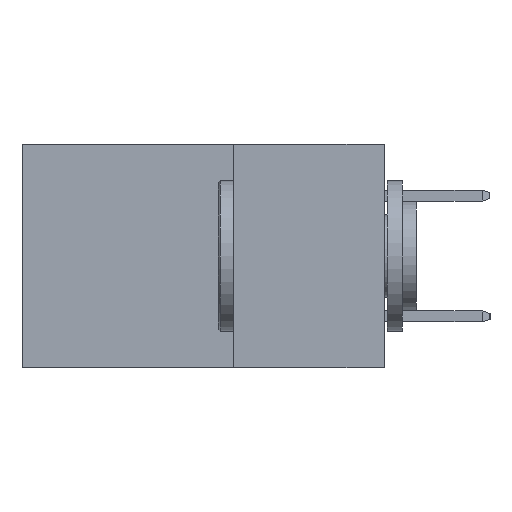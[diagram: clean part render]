
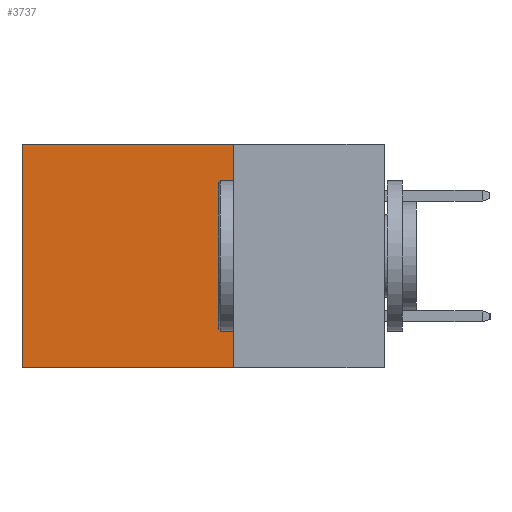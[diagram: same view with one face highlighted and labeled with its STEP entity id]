
A CAD part, left-side view. The second image highlights one B-rep face of the part: STEP entity #3737.
In plain terms, the highlighted planar face has unit normal (-1, 0, 0).
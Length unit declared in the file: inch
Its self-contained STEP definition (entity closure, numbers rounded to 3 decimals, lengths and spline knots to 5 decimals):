
#988 = EDGE_CURVE ( 'NONE', #3144, #2334, #13684, .T. ) ;
#1966 = EDGE_CURVE ( 'NONE', #3286, #10497, #11336, .T. ) ;
#2065 = VECTOR ( 'NONE', #4702, 39.37008 ) ;
#2334 = VERTEX_POINT ( 'NONE', #8466 ) ;
#2817 = FACE_OUTER_BOUND ( 'NONE', #7623, .T. ) ;
#3045 = DIRECTION ( 'NONE',  ( 0., 0., -1. ) ) ;
#3144 = VERTEX_POINT ( 'NONE', #10999 ) ;
#3286 = VERTEX_POINT ( 'NONE', #6830 ) ;
#3434 = CARTESIAN_POINT ( 'NONE',  ( 0.2615, 0.6, -0.37 ) ) ;
#3737 = ADVANCED_FACE ( 'NONE', ( #2817 ), #5657, .F. ) ;
#3754 = AXIS2_PLACEMENT_3D ( 'NONE', #6636, #5295, #5189 ) ;
#4532 = CARTESIAN_POINT ( 'NONE',  ( 0.2615, 0.25, 0. ) ) ;
#4702 = DIRECTION ( 'NONE',  ( 0., 1., 0. ) ) ;
#5082 = LINE ( 'NONE', #15346, #11401 ) ;
#5189 = DIRECTION ( 'NONE',  ( 0., 0., -1. ) ) ;
#5295 = DIRECTION ( 'NONE',  ( 1., 0., 0. ) ) ;
#5657 = PLANE ( 'NONE',  #3754 ) ;
#5928 = ORIENTED_EDGE ( 'NONE', *, *, #1966, .T. ) ;
#5994 = VECTOR ( 'NONE', #3045, 39.37008 ) ;
#6386 = EDGE_CURVE ( 'NONE', #10497, #2334, #9890, .T. ) ;
#6636 = CARTESIAN_POINT ( 'NONE',  ( 0.2615, 0.25, -0.37 ) ) ;
#6830 = CARTESIAN_POINT ( 'NONE',  ( 0.2615, 0.25, 0. ) ) ;
#7246 = CARTESIAN_POINT ( 'NONE',  ( 0.2615, 0.6, 0. ) ) ;
#7623 = EDGE_LOOP ( 'NONE', ( #9704, #14377, #8289, #5928 ) ) ;
#8035 = CARTESIAN_POINT ( 'NONE',  ( 0.2615, 0.25, -0.37 ) ) ;
#8289 = ORIENTED_EDGE ( 'NONE', *, *, #11616, .F. ) ;
#8439 = DIRECTION ( 'NONE',  ( 0., 1., 0. ) ) ;
#8466 = CARTESIAN_POINT ( 'NONE',  ( 0.2615, 0.6, -0.37 ) ) ;
#9704 = ORIENTED_EDGE ( 'NONE', *, *, #6386, .T. ) ;
#9890 = LINE ( 'NONE', #3434, #5994 ) ;
#10497 = VERTEX_POINT ( 'NONE', #7246 ) ;
#10618 = VECTOR ( 'NONE', #8439, 39.37008 ) ;
#10999 = CARTESIAN_POINT ( 'NONE',  ( 0.2615, 0.25, -0.37 ) ) ;
#11336 = LINE ( 'NONE', #4532, #2065 ) ;
#11401 = VECTOR ( 'NONE', #15258, 39.37008 ) ;
#11616 = EDGE_CURVE ( 'NONE', #3286, #3144, #5082, .T. ) ;
#13684 = LINE ( 'NONE', #8035, #10618 ) ;
#14377 = ORIENTED_EDGE ( 'NONE', *, *, #988, .F. ) ;
#15258 = DIRECTION ( 'NONE',  ( 0., 0., -1. ) ) ;
#15346 = CARTESIAN_POINT ( 'NONE',  ( 0.2615, 0.25, -0.37 ) ) ;
